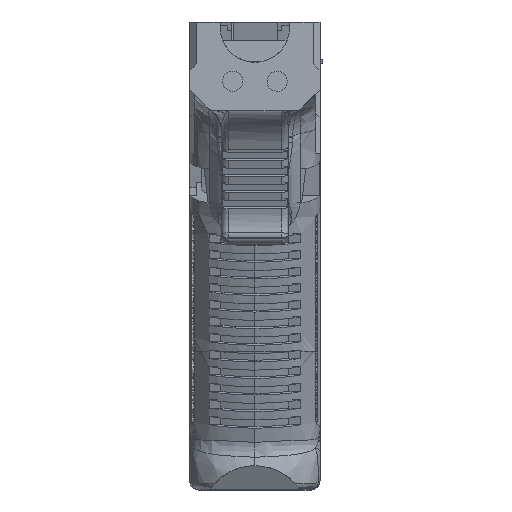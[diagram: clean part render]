
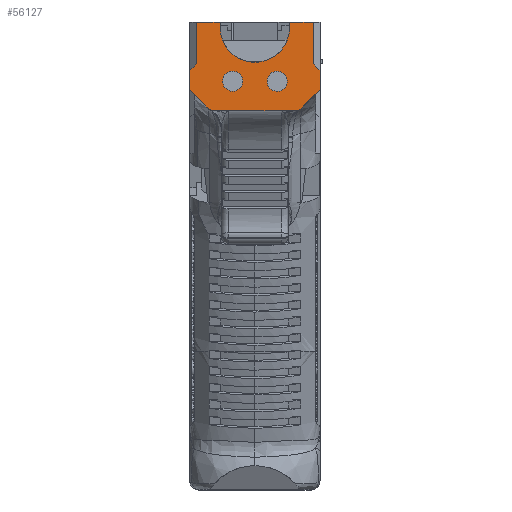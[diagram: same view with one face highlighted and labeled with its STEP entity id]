
A CAD part, left-side view. The second image highlights one B-rep face of the part: STEP entity #56127.
In plain terms, the highlighted planar face has unit normal (-1, 0, 0).
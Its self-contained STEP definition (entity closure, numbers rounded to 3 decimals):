
#7304=FACE_BOUND('',#12161,.T.);
#7305=FACE_BOUND('',#12162,.T.);
#7730=PLANE('',#59527);
#8768=FACE_OUTER_BOUND('',#12160,.T.);
#12160=EDGE_LOOP('',(#38293,#38294,#38295,#38296,#38297,#38298,#38299,#38300,
#38301,#38302,#38303,#38304,#38305,#38306,#38307,#38308));
#12161=EDGE_LOOP('',(#38309));
#12162=EDGE_LOOP('',(#38310));
#16002=LINE('',#67267,#19642);
#16003=LINE('',#67269,#19643);
#16004=LINE('',#67271,#19644);
#16005=LINE('',#67273,#19645);
#16006=LINE('',#67275,#19646);
#16007=LINE('',#67277,#19647);
#16008=LINE('',#67281,#19648);
#16009=LINE('',#67285,#19649);
#16010=LINE('',#67287,#19650);
#16011=LINE('',#67289,#19651);
#16012=LINE('',#67291,#19652);
#16013=LINE('',#67293,#19653);
#16014=LINE('',#67294,#19654);
#19642=VECTOR('',#60905,10.);
#19643=VECTOR('',#60906,10.);
#19644=VECTOR('',#60907,10.);
#19645=VECTOR('',#60908,10.);
#19646=VECTOR('',#60909,10.);
#19647=VECTOR('',#60910,10.);
#19648=VECTOR('',#60913,10.);
#19649=VECTOR('',#60916,10.);
#19650=VECTOR('',#60917,10.);
#19651=VECTOR('',#60918,10.);
#19652=VECTOR('',#60919,10.);
#19653=VECTOR('',#60920,10.);
#19654=VECTOR('',#60921,10.);
#23282=CIRCLE('',#59528,7.765);
#23283=CIRCLE('',#59529,3.);
#23284=CIRCLE('',#59530,3.);
#23285=CIRCLE('',#59531,2.25);
#23286=CIRCLE('',#59532,2.25);
#23506=VERTEX_POINT('',#67263);
#23507=VERTEX_POINT('',#67264);
#23508=VERTEX_POINT('',#67266);
#23509=VERTEX_POINT('',#67268);
#23510=VERTEX_POINT('',#67270);
#23511=VERTEX_POINT('',#67272);
#23512=VERTEX_POINT('',#67274);
#23513=VERTEX_POINT('',#67276);
#23514=VERTEX_POINT('',#67278);
#23515=VERTEX_POINT('',#67280);
#23516=VERTEX_POINT('',#67282);
#23517=VERTEX_POINT('',#67284);
#23518=VERTEX_POINT('',#67286);
#23519=VERTEX_POINT('',#67288);
#23520=VERTEX_POINT('',#67290);
#23521=VERTEX_POINT('',#67292);
#23522=VERTEX_POINT('',#67295);
#23523=VERTEX_POINT('',#67297);
#29398=EDGE_CURVE('',#23506,#23507,#23282,.T.);
#29399=EDGE_CURVE('',#23506,#23508,#16002,.T.);
#29400=EDGE_CURVE('',#23508,#23509,#16003,.T.);
#29401=EDGE_CURVE('',#23509,#23510,#16004,.T.);
#29402=EDGE_CURVE('',#23510,#23511,#16005,.T.);
#29403=EDGE_CURVE('',#23511,#23512,#16006,.T.);
#29404=EDGE_CURVE('',#23512,#23513,#16007,.T.);
#29405=EDGE_CURVE('',#23513,#23514,#23283,.T.);
#29406=EDGE_CURVE('',#23514,#23515,#16008,.T.);
#29407=EDGE_CURVE('',#23515,#23516,#23284,.T.);
#29408=EDGE_CURVE('',#23516,#23517,#16009,.T.);
#29409=EDGE_CURVE('',#23517,#23518,#16010,.T.);
#29410=EDGE_CURVE('',#23518,#23519,#16011,.T.);
#29411=EDGE_CURVE('',#23519,#23520,#16012,.T.);
#29412=EDGE_CURVE('',#23520,#23521,#16013,.T.);
#29413=EDGE_CURVE('',#23521,#23507,#16014,.T.);
#29414=EDGE_CURVE('',#23522,#23522,#23285,.T.);
#29415=EDGE_CURVE('',#23523,#23523,#23286,.T.);
#38293=ORIENTED_EDGE('',*,*,#29398,.F.);
#38294=ORIENTED_EDGE('',*,*,#29399,.T.);
#38295=ORIENTED_EDGE('',*,*,#29400,.T.);
#38296=ORIENTED_EDGE('',*,*,#29401,.T.);
#38297=ORIENTED_EDGE('',*,*,#29402,.T.);
#38298=ORIENTED_EDGE('',*,*,#29403,.T.);
#38299=ORIENTED_EDGE('',*,*,#29404,.T.);
#38300=ORIENTED_EDGE('',*,*,#29405,.T.);
#38301=ORIENTED_EDGE('',*,*,#29406,.T.);
#38302=ORIENTED_EDGE('',*,*,#29407,.T.);
#38303=ORIENTED_EDGE('',*,*,#29408,.T.);
#38304=ORIENTED_EDGE('',*,*,#29409,.T.);
#38305=ORIENTED_EDGE('',*,*,#29410,.T.);
#38306=ORIENTED_EDGE('',*,*,#29411,.T.);
#38307=ORIENTED_EDGE('',*,*,#29412,.T.);
#38308=ORIENTED_EDGE('',*,*,#29413,.T.);
#38309=ORIENTED_EDGE('',*,*,#29414,.T.);
#38310=ORIENTED_EDGE('',*,*,#29415,.T.);
#56127=ADVANCED_FACE('',(#8768,#7304,#7305),#7730,.F.);
#59527=AXIS2_PLACEMENT_3D('',#67262,#60901,#60902);
#59528=AXIS2_PLACEMENT_3D('',#67265,#60903,#60904);
#59529=AXIS2_PLACEMENT_3D('',#67279,#60911,#60912);
#59530=AXIS2_PLACEMENT_3D('',#67283,#60914,#60915);
#59531=AXIS2_PLACEMENT_3D('',#67296,#60922,#60923);
#59532=AXIS2_PLACEMENT_3D('',#67298,#60924,#60925);
#60901=DIRECTION('center_axis',(1.,0.,0.));
#60902=DIRECTION('ref_axis',(0.,1.,0.));
#60903=DIRECTION('center_axis',(-1.,0.,0.));
#60904=DIRECTION('ref_axis',(0.,0.,
-1.));
#60905=DIRECTION('',(0.,0.,1.));
#60906=DIRECTION('',(0.,1.,0.));
#60907=DIRECTION('',(0.,0.,-1.));
#60908=DIRECTION('',(0.,0.707,-0.707));
#60909=DIRECTION('',(0.,0.,-1.));
#60910=DIRECTION('',(0.,-0.707,-0.707));
#60911=DIRECTION('center_axis',(-1.,0.,0.));
#60912=DIRECTION('ref_axis',(0.,0.383,-0.924));
#60913=DIRECTION('',(0.,-1.,0.));
#60914=DIRECTION('center_axis',(-1.,0.,0.));
#60915=DIRECTION('ref_axis',(0.,-0.383,-0.924));
#60916=DIRECTION('',(0.,-0.707,0.707));
#60917=DIRECTION('',(0.,0.,1.));
#60918=DIRECTION('',(0.,0.707,0.707));
#60919=DIRECTION('',(0.,0.,1.));
#60920=DIRECTION('',(0.,1.,0.));
#60921=DIRECTION('',(0.,0.,-1.));
#60922=DIRECTION('center_axis',(1.,0.,0.));
#60923=DIRECTION('ref_axis',(0.,1.,0.));
#60924=DIRECTION('center_axis',(1.,0.,0.));
#60925=DIRECTION('ref_axis',(0.,0.726,-0.688));
#67262=CARTESIAN_POINT('Origin',(237.489,26.849,-196.648));
#67263=CARTESIAN_POINT('',(237.489,34.614,-145.477));
#67264=CARTESIAN_POINT('',(237.489,19.086,-145.477));
#67265=CARTESIAN_POINT('Origin',(237.489,26.85,-145.35));
#67266=CARTESIAN_POINT('',(237.489,34.614,-144.061));
#67267=CARTESIAN_POINT('',(237.489,34.614,-170.936));
#67268=CARTESIAN_POINT('',(237.489,39.966,-144.061));
#67269=CARTESIAN_POINT('',(237.489,19.237,-144.061));
#67270=CARTESIAN_POINT('',(237.489,39.966,-153.447));
#67271=CARTESIAN_POINT('',(237.489,39.966,-170.048));
#67272=CARTESIAN_POINT('',(237.489,41.466,-154.947));
#67273=CARTESIAN_POINT('',(237.489,47.862,-161.343));
#67274=CARTESIAN_POINT('',(237.489,41.466,-159.25));
#67275=CARTESIAN_POINT('',(237.489,41.466,-170.301));
#67276=CARTESIAN_POINT('',(237.489,37.595,-163.122));
#67277=CARTESIAN_POINT('',(237.489,27.275,-173.442));
#67278=CARTESIAN_POINT('',(237.489,35.473,-164.));
#67279=CARTESIAN_POINT('Origin',(237.489,35.473,-161.));
#67280=CARTESIAN_POINT('',(237.489,18.227,-164.));
#67281=CARTESIAN_POINT('',(237.489,26.85,-164.));
#67282=CARTESIAN_POINT('',(237.489,16.105,-163.122));
#67283=CARTESIAN_POINT('Origin',(237.489,18.227,-161.));
#67284=CARTESIAN_POINT('',(237.489,12.234,-159.25));
#67285=CARTESIAN_POINT('',(237.489,26.425,-173.441));
#67286=CARTESIAN_POINT('',(237.489,12.234,-154.947));
#67287=CARTESIAN_POINT('',(237.489,12.234,-170.301));
#67288=CARTESIAN_POINT('',(237.489,13.734,-153.447));
#67289=CARTESIAN_POINT('',(237.489,5.837,-161.343));
#67290=CARTESIAN_POINT('',(237.489,13.734,-144.061));
#67291=CARTESIAN_POINT('',(237.489,13.734,-175.048));
#67292=CARTESIAN_POINT('',(237.489,19.086,-144.061));
#67293=CARTESIAN_POINT('',(237.489,19.237,-144.061));
#67294=CARTESIAN_POINT('',(237.489,19.086,-170.936));
#67295=CARTESIAN_POINT('',(237.489,29.6,-157.346));
#67296=CARTESIAN_POINT('Origin',(237.489,31.85,-157.346));
#67297=CARTESIAN_POINT('',(237.489,20.217,-155.798));
#67298=CARTESIAN_POINT('Origin',(237.489,21.85,-157.346));
